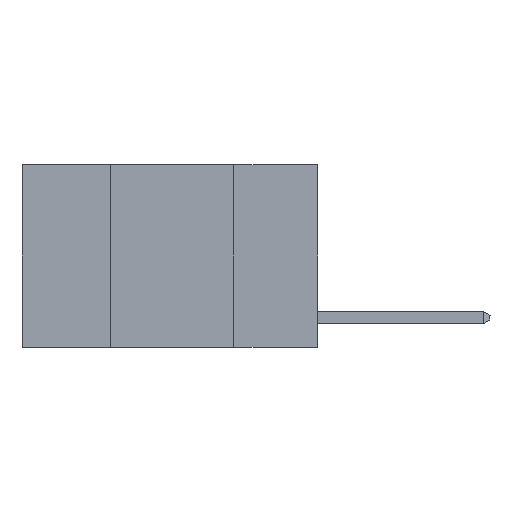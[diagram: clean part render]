
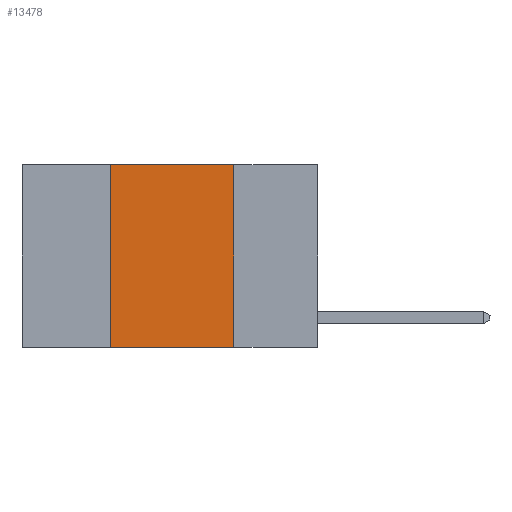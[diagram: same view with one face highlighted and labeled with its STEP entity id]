
A CAD part, left-side view. The second image highlights one B-rep face of the part: STEP entity #13478.
In plain terms, the highlighted planar face has unit normal (-1, 0, 0).
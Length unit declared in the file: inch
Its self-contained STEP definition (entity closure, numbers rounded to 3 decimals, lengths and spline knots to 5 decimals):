
#1732 = DIRECTION ( 'NONE',  ( 0., -1., 0. ) ) ;
#2640 = CARTESIAN_POINT ( 'NONE',  ( 0., 0.17, 0. ) ) ;
#3654 = CARTESIAN_POINT ( 'NONE',  ( 0., 0.6, 0. ) ) ;
#4098 = VECTOR ( 'NONE', #10967, 39.37008 ) ;
#4179 = AXIS2_PLACEMENT_3D ( 'NONE', #3654, #16986, #5578 ) ;
#4657 = EDGE_LOOP ( 'NONE', ( #23354, #14365, #13789, #4798 ) ) ;
#4798 = ORIENTED_EDGE ( 'NONE', *, *, #8780, .T. ) ;
#5241 = DIRECTION ( 'NONE',  ( 0., 0., 1. ) ) ;
#5578 = DIRECTION ( 'NONE',  ( 0., 0., -1. ) ) ;
#8106 = EDGE_CURVE ( 'NONE', #23421, #20953, #14849, .T. ) ;
#8780 = EDGE_CURVE ( 'NONE', #12519, #15574, #13954, .T. ) ;
#8860 = VECTOR ( 'NONE', #1732, 39.37008 ) ;
#9221 = CARTESIAN_POINT ( 'NONE',  ( 0., 0.42, 0. ) ) ;
#10008 = FACE_OUTER_BOUND ( 'NONE', #4657, .T. ) ;
#10299 = CARTESIAN_POINT ( 'NONE',  ( 0., 0.42, -0.37 ) ) ;
#10967 = DIRECTION ( 'NONE',  ( 0., -1., 0. ) ) ;
#11074 = LINE ( 'NONE', #2640, #16133 ) ;
#12519 = VERTEX_POINT ( 'NONE', #10299 ) ;
#12818 = CARTESIAN_POINT ( 'NONE',  ( 0., 0.17, 0. ) ) ;
#13176 = PLANE ( 'NONE',  #4179 ) ;
#13202 = CARTESIAN_POINT ( 'NONE',  ( 0., 0.6, -0.37 ) ) ;
#13478 = ADVANCED_FACE ( 'NONE', ( #10008 ), #13176, .F. ) ;
#13789 = ORIENTED_EDGE ( 'NONE', *, *, #24612, .F. ) ;
#13954 = LINE ( 'NONE', #13202, #8860 ) ;
#14365 = ORIENTED_EDGE ( 'NONE', *, *, #8106, .F. ) ;
#14581 = VECTOR ( 'NONE', #5241, 39.37008 ) ;
#14849 = LINE ( 'NONE', #24350, #4098 ) ;
#15574 = VERTEX_POINT ( 'NONE', #21785 ) ;
#16008 = DIRECTION ( 'NONE',  ( 0., 0., -1. ) ) ;
#16133 = VECTOR ( 'NONE', #16008, 39.37008 ) ;
#16986 = DIRECTION ( 'NONE',  ( 1., 0., 0. ) ) ;
#18519 = CARTESIAN_POINT ( 'NONE',  ( 0., 0.42, 0. ) ) ;
#20246 = LINE ( 'NONE', #18519, #14581 ) ;
#20953 = VERTEX_POINT ( 'NONE', #12818 ) ;
#21785 = CARTESIAN_POINT ( 'NONE',  ( 0., 0.17, -0.37 ) ) ;
#22059 = EDGE_CURVE ( 'NONE', #20953, #15574, #11074, .T. ) ;
#23354 = ORIENTED_EDGE ( 'NONE', *, *, #22059, .F. ) ;
#23421 = VERTEX_POINT ( 'NONE', #9221 ) ;
#24350 = CARTESIAN_POINT ( 'NONE',  ( 0., 0.6, 0. ) ) ;
#24612 = EDGE_CURVE ( 'NONE', #12519, #23421, #20246, .T. ) ;
